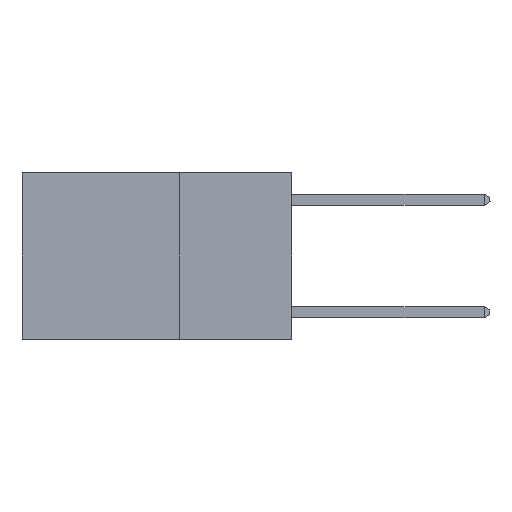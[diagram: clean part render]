
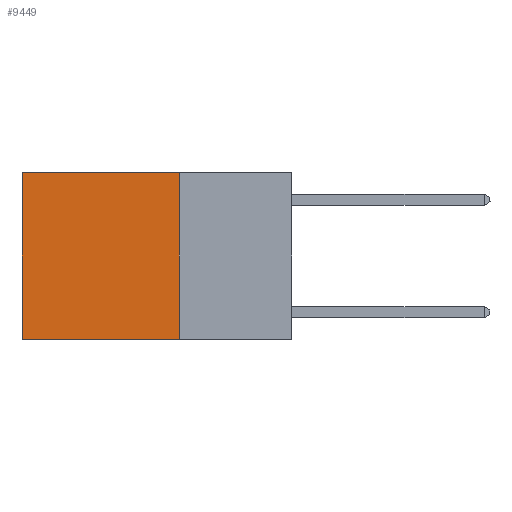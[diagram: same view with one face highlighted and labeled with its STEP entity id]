
A CAD part, left-side view. The second image highlights one B-rep face of the part: STEP entity #9449.
In plain terms, the highlighted planar face has unit normal (-1, 0, 0).
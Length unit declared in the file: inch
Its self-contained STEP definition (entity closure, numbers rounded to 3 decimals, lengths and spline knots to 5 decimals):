
#62 = VECTOR ( 'NONE', #6354, 39.37008 ) ;
#141 = EDGE_CURVE ( 'NONE', #2617, #2313, #2501, .T. ) ;
#648 = FACE_OUTER_BOUND ( 'NONE', #4333, .T. ) ;
#827 = PLANE ( 'NONE',  #6480 ) ;
#841 = ORIENTED_EDGE ( 'NONE', *, *, #6992, .T. ) ;
#1414 = LINE ( 'NONE', #1422, #9304 ) ;
#1422 = CARTESIAN_POINT ( 'NONE',  ( 0.2625, 0.6, 0. ) ) ;
#1762 = CARTESIAN_POINT ( 'NONE',  ( 0.2625, 0.25, 0. ) ) ;
#2313 = VERTEX_POINT ( 'NONE', #8447 ) ;
#2335 = CARTESIAN_POINT ( 'NONE',  ( 0.2625, 0.25, 0. ) ) ;
#2501 = LINE ( 'NONE', #10086, #62 ) ;
#2617 = VERTEX_POINT ( 'NONE', #10196 ) ;
#2634 = DIRECTION ( 'NONE',  ( 0., 0., -1. ) ) ;
#2823 = DIRECTION ( 'NONE',  ( 0., 0., -1. ) ) ;
#3034 = CARTESIAN_POINT ( 'NONE',  ( 0.2625, 0.25, 0. ) ) ;
#3596 = LINE ( 'NONE', #2335, #5672 ) ;
#4333 = EDGE_LOOP ( 'NONE', ( #841, #8236, #9262, #7086 ) ) ;
#5288 = EDGE_CURVE ( 'NONE', #5999, #9825, #3596, .T. ) ;
#5623 = VECTOR ( 'NONE', #2823, 39.37008 ) ;
#5672 = VECTOR ( 'NONE', #7029, 39.37008 ) ;
#5999 = VERTEX_POINT ( 'NONE', #3034 ) ;
#6354 = DIRECTION ( 'NONE',  ( 0., 1., 0. ) ) ;
#6480 = AXIS2_PLACEMENT_3D ( 'NONE', #1762, #7310, #2634 ) ;
#6717 = CARTESIAN_POINT ( 'NONE',  ( 0.2625, 0.25, 0. ) ) ;
#6992 = EDGE_CURVE ( 'NONE', #9825, #2313, #1414, .T. ) ;
#7029 = DIRECTION ( 'NONE',  ( 0., 1., 0. ) ) ;
#7086 = ORIENTED_EDGE ( 'NONE', *, *, #5288, .T. ) ;
#7310 = DIRECTION ( 'NONE',  ( 1., 0., 0. ) ) ;
#7807 = DIRECTION ( 'NONE',  ( 0., 0., -1. ) ) ;
#8236 = ORIENTED_EDGE ( 'NONE', *, *, #141, .F. ) ;
#8447 = CARTESIAN_POINT ( 'NONE',  ( 0.2625, 0.6, -0.37 ) ) ;
#8958 = EDGE_CURVE ( 'NONE', #5999, #2617, #9853, .T. ) ;
#9121 = CARTESIAN_POINT ( 'NONE',  ( 0.2625, 0.6, 0. ) ) ;
#9262 = ORIENTED_EDGE ( 'NONE', *, *, #8958, .F. ) ;
#9304 = VECTOR ( 'NONE', #7807, 39.37008 ) ;
#9449 = ADVANCED_FACE ( 'NONE', ( #648 ), #827, .F. ) ;
#9825 = VERTEX_POINT ( 'NONE', #9121 ) ;
#9853 = LINE ( 'NONE', #6717, #5623 ) ;
#10086 = CARTESIAN_POINT ( 'NONE',  ( 0.2625, 0.25, -0.37 ) ) ;
#10196 = CARTESIAN_POINT ( 'NONE',  ( 0.2625, 0.25, -0.37 ) ) ;
